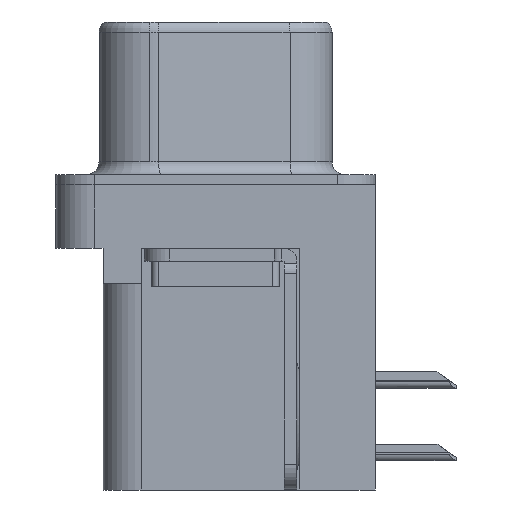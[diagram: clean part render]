
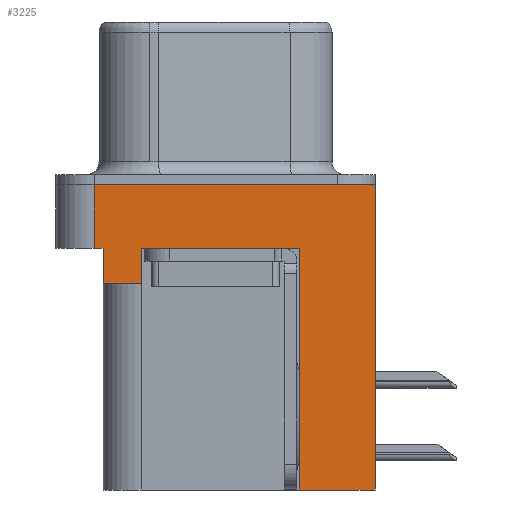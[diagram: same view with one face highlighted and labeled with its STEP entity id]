
A CAD part, left-side view. The second image highlights one B-rep face of the part: STEP entity #3225.
In plain terms, the highlighted planar face has unit normal (-1, 0, 0).
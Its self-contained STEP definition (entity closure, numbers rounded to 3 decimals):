
#571 = EDGE_CURVE ( 'NONE', #1478, #13639, #7032, .T. ) ;
#762 = VECTOR ( 'NONE', #20130, 1000. ) ;
#799 = PLANE ( 'NONE',  #18762 ) ;
#1000 = LINE ( 'NONE', #3435, #12660 ) ;
#1404 = VECTOR ( 'NONE', #3110, 1000. ) ;
#1478 = VERTEX_POINT ( 'NONE', #13313 ) ;
#1628 = EDGE_CURVE ( 'NONE', #14195, #6521, #9779, .T. ) ;
#1771 = CARTESIAN_POINT ( 'NONE',  ( -3., -3.295, -2.5 ) ) ;
#2920 = DIRECTION ( 'NONE',  ( -1., 0., 0. ) ) ;
#3110 = DIRECTION ( 'NONE',  ( 0., 0., 1. ) ) ;
#3170 = LINE ( 'NONE', #12718, #13061 ) ;
#3225 = ADVANCED_FACE ( 'NONE', ( #5654 ), #799, .T. ) ;
#3378 = CARTESIAN_POINT ( 'NONE',  ( -3., -3.295, -12. ) ) ;
#3435 = CARTESIAN_POINT ( 'NONE',  ( -3., -6.275, 0. ) ) ;
#3973 = EDGE_LOOP ( 'NONE', ( #18712, #21175, #23800, #16753, #13821, #7366, #21395, #16299, #16419, #9441 ) ) ;
#4082 = CARTESIAN_POINT ( 'NONE',  ( -3., 4.775, 0. ) ) ;
#4296 = LINE ( 'NONE', #7558, #7490 ) ;
#4317 = LINE ( 'NONE', #17300, #11442 ) ;
#4429 = VERTEX_POINT ( 'NONE', #1771 ) ;
#5654 = FACE_OUTER_BOUND ( 'NONE', #3973, .T. ) ;
#6105 = LINE ( 'NONE', #3378, #10796 ) ;
#6119 = CARTESIAN_POINT ( 'NONE',  ( -3., 2.895, -2.5 ) ) ;
#6133 = VERTEX_POINT ( 'NONE', #6119 ) ;
#6521 = VERTEX_POINT ( 'NONE', #4082 ) ;
#6537 = VERTEX_POINT ( 'NONE', #11494 ) ;
#6705 = EDGE_CURVE ( 'NONE', #6133, #4429, #23002, .T. ) ;
#6911 = EDGE_CURVE ( 'NONE', #19253, #4429, #14257, .T. ) ;
#7032 = LINE ( 'NONE', #22165, #17551 ) ;
#7123 = DIRECTION ( 'NONE',  ( 0., -1., 0. ) ) ;
#7340 = VERTEX_POINT ( 'NONE', #20383 ) ;
#7366 = ORIENTED_EDGE ( 'NONE', *, *, #22008, .T. ) ;
#7490 = VECTOR ( 'NONE', #11473, 1000. ) ;
#7558 = CARTESIAN_POINT ( 'NONE',  ( -3., -6.275, -2.5 ) ) ;
#8148 = CARTESIAN_POINT ( 'NONE',  ( -3., 4.775, -2.5 ) ) ;
#9031 = CARTESIAN_POINT ( 'NONE',  ( -3., -3.295, -12. ) ) ;
#9216 = EDGE_CURVE ( 'NONE', #6521, #13639, #1000, .T. ) ;
#9441 = ORIENTED_EDGE ( 'NONE', *, *, #571, .T. ) ;
#9779 = LINE ( 'NONE', #16314, #762 ) ;
#10741 = DIRECTION ( 'NONE',  ( 0., 0., 1. ) ) ;
#10796 = VECTOR ( 'NONE', #14445, 1000. ) ;
#11442 = VECTOR ( 'NONE', #21538, 1000. ) ;
#11473 = DIRECTION ( 'NONE',  ( 0., -1., 0. ) ) ;
#11494 = CARTESIAN_POINT ( 'NONE',  ( -3., 4.425, -3.9 ) ) ;
#12349 = CARTESIAN_POINT ( 'NONE',  ( -3., -6.275, 0. ) ) ;
#12660 = VECTOR ( 'NONE', #23884, 1000. ) ;
#12718 = CARTESIAN_POINT ( 'NONE',  ( -3., 4.425, -3.9 ) ) ;
#12888 = EDGE_CURVE ( 'NONE', #1478, #19253, #6105, .T. ) ;
#13059 = EDGE_CURVE ( 'NONE', #6537, #15626, #19552, .T. ) ;
#13061 = VECTOR ( 'NONE', #21795, 1000. ) ;
#13313 = CARTESIAN_POINT ( 'NONE',  ( -3., -6.275, -12. ) ) ;
#13639 = VERTEX_POINT ( 'NONE', #12349 ) ;
#13821 = ORIENTED_EDGE ( 'NONE', *, *, #15378, .F. ) ;
#13847 = CARTESIAN_POINT ( 'NONE',  ( -3., -6.275, -2.5 ) ) ;
#14080 = DIRECTION ( 'NONE',  ( 0., 0., 1. ) ) ;
#14195 = VERTEX_POINT ( 'NONE', #8148 ) ;
#14257 = LINE ( 'NONE', #21436, #1404 ) ;
#14445 = DIRECTION ( 'NONE',  ( 0., 1., 0. ) ) ;
#15378 = EDGE_CURVE ( 'NONE', #7340, #6537, #3170, .T. ) ;
#15626 = VERTEX_POINT ( 'NONE', #16581 ) ;
#15734 = EDGE_CURVE ( 'NONE', #14195, #15626, #4296, .T. ) ;
#16299 = ORIENTED_EDGE ( 'NONE', *, *, #6911, .F. ) ;
#16314 = CARTESIAN_POINT ( 'NONE',  ( -3., 4.775, -2.5 ) ) ;
#16419 = ORIENTED_EDGE ( 'NONE', *, *, #12888, .F. ) ;
#16581 = CARTESIAN_POINT ( 'NONE',  ( -3., 4.425, -2.5 ) ) ;
#16753 = ORIENTED_EDGE ( 'NONE', *, *, #13059, .F. ) ;
#16821 = VECTOR ( 'NONE', #7123, 1000. ) ;
#16903 = VECTOR ( 'NONE', #10741, 1000. ) ;
#17300 = CARTESIAN_POINT ( 'NONE',  ( -3., 2.895, -3.9 ) ) ;
#17551 = VECTOR ( 'NONE', #18498, 1000. ) ;
#18498 = DIRECTION ( 'NONE',  ( 0., 0., 1. ) ) ;
#18712 = ORIENTED_EDGE ( 'NONE', *, *, #9216, .F. ) ;
#18762 = AXIS2_PLACEMENT_3D ( 'NONE', #13847, #2920, #14080 ) ;
#19253 = VERTEX_POINT ( 'NONE', #9031 ) ;
#19552 = LINE ( 'NONE', #21768, #16903 ) ;
#20130 = DIRECTION ( 'NONE',  ( 0., 0., 1. ) ) ;
#20383 = CARTESIAN_POINT ( 'NONE',  ( -3., 2.895, -3.9 ) ) ;
#21175 = ORIENTED_EDGE ( 'NONE', *, *, #1628, .F. ) ;
#21395 = ORIENTED_EDGE ( 'NONE', *, *, #6705, .T. ) ;
#21436 = CARTESIAN_POINT ( 'NONE',  ( -3., -3.295, -12. ) ) ;
#21538 = DIRECTION ( 'NONE',  ( 0., 0., 1. ) ) ;
#21768 = CARTESIAN_POINT ( 'NONE',  ( -3., 4.425, -3.9 ) ) ;
#21795 = DIRECTION ( 'NONE',  ( 0., 1., 0. ) ) ;
#22008 = EDGE_CURVE ( 'NONE', #7340, #6133, #4317, .T. ) ;
#22165 = CARTESIAN_POINT ( 'NONE',  ( -3., -6.275, -2.5 ) ) ;
#22212 = CARTESIAN_POINT ( 'NONE',  ( -3., -6.275, -2.5 ) ) ;
#23002 = LINE ( 'NONE', #22212, #16821 ) ;
#23800 = ORIENTED_EDGE ( 'NONE', *, *, #15734, .T. ) ;
#23884 = DIRECTION ( 'NONE',  ( 0., -1., 0. ) ) ;
